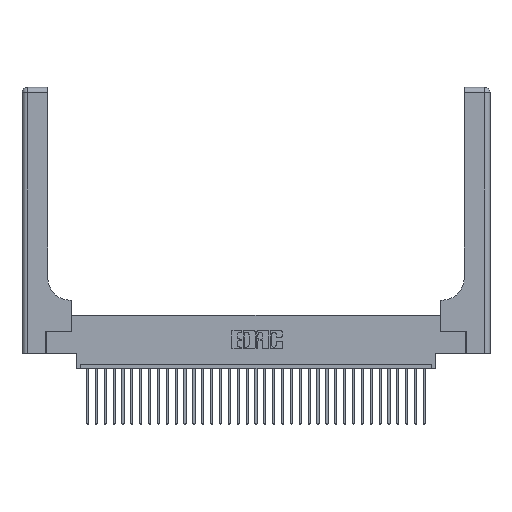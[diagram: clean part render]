
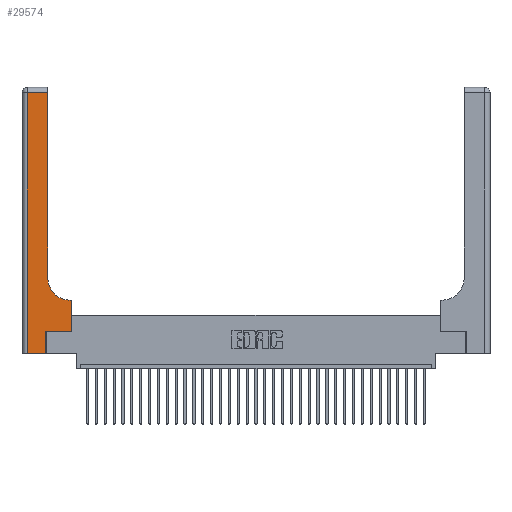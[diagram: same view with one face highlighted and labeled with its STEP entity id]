
A CAD part, top view. The second image highlights one B-rep face of the part: STEP entity #29574.
In plain terms, the highlighted planar face has unit normal (0, 0, 1).
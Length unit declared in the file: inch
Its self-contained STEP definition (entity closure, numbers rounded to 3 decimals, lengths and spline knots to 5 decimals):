
#1807 = VECTOR ( 'NONE', #23549, 39.37008 ) ;
#2154 = VERTEX_POINT ( 'NONE', #17191 ) ;
#2753 = CIRCLE ( 'NONE', #10083, 0.25 ) ;
#4222 = CARTESIAN_POINT ( 'NONE',  ( 0.2915, 3., 0.37 ) ) ;
#4265 = EDGE_CURVE ( 'NONE', #19982, #17829, #9771, .T. ) ;
#4856 = VERTEX_POINT ( 'NONE', #8780 ) ;
#5241 = VECTOR ( 'NONE', #5458, 39.37008 ) ;
#5458 = DIRECTION ( 'NONE',  ( 0., -1., 0. ) ) ;
#6608 = CARTESIAN_POINT ( 'NONE',  ( 0., 3., 0.37 ) ) ;
#6723 = CARTESIAN_POINT ( 'NONE',  ( 0.269, 0., 0.37 ) ) ;
#7131 = FACE_OUTER_BOUND ( 'NONE', #16927, .T. ) ;
#7163 = CARTESIAN_POINT ( 'NONE',  ( 0.269, 0.25, 0.37 ) ) ;
#7577 = VERTEX_POINT ( 'NONE', #15437 ) ;
#8157 = DIRECTION ( 'NONE',  ( 1., 0., 0. ) ) ;
#8568 = LINE ( 'NONE', #16224, #1807 ) ;
#8780 = CARTESIAN_POINT ( 'NONE',  ( 0.06, 2.94, 0.37 ) ) ;
#9764 = EDGE_CURVE ( 'NONE', #7577, #31835, #14838, .T. ) ;
#9771 = LINE ( 'NONE', #4222, #22392 ) ;
#9813 = ORIENTED_EDGE ( 'NONE', *, *, #4265, .T. ) ;
#9881 = ORIENTED_EDGE ( 'NONE', *, *, #16773, .T. ) ;
#10083 = AXIS2_PLACEMENT_3D ( 'NONE', #32426, #24241, #8157 ) ;
#11196 = ORIENTED_EDGE ( 'NONE', *, *, #32418, .T. ) ;
#11605 = VECTOR ( 'NONE', #15889, 39.37008 ) ;
#11642 = CARTESIAN_POINT ( 'NONE',  ( 0.5585, 0.25, 0.37 ) ) ;
#11694 = CARTESIAN_POINT ( 'NONE',  ( 0.5415, 0.6, 0.37 ) ) ;
#12019 = EDGE_CURVE ( 'NONE', #17829, #4856, #26405, .T. ) ;
#12811 = AXIS2_PLACEMENT_3D ( 'NONE', #6608, #15139, #17930 ) ;
#12861 = ORIENTED_EDGE ( 'NONE', *, *, #9764, .T. ) ;
#14224 = LINE ( 'NONE', #33709, #27313 ) ;
#14408 = VERTEX_POINT ( 'NONE', #31009 ) ;
#14838 = LINE ( 'NONE', #7163, #24172 ) ;
#15139 = DIRECTION ( 'NONE',  ( 0., 0., -1. ) ) ;
#15437 = CARTESIAN_POINT ( 'NONE',  ( 0.269, 0.25, 0.37 ) ) ;
#15889 = DIRECTION ( 'NONE',  ( -1., 0., 0. ) ) ;
#15929 = CARTESIAN_POINT ( 'NONE',  ( 0.2915, 0.85, 0.37 ) ) ;
#16224 = CARTESIAN_POINT ( 'NONE',  ( 0.2915, 0.6, 0.37 ) ) ;
#16773 = EDGE_CURVE ( 'NONE', #14408, #25531, #8568, .T. ) ;
#16927 = EDGE_LOOP ( 'NONE', ( #9813, #30972, #29127, #30011, #11196, #12861, #18598, #9881, #34941 ) ) ;
#17075 = VECTOR ( 'NONE', #30479, 39.37008 ) ;
#17191 = CARTESIAN_POINT ( 'NONE',  ( 0.269, 0., 0.37 ) ) ;
#17829 = VERTEX_POINT ( 'NONE', #33732 ) ;
#17930 = DIRECTION ( 'NONE',  ( -1., 0., 0. ) ) ;
#18349 = CARTESIAN_POINT ( 'NONE',  ( 0., 2.94, 0.37 ) ) ;
#18381 = DIRECTION ( 'NONE',  ( 0., 1., 0. ) ) ;
#18598 = ORIENTED_EDGE ( 'NONE', *, *, #21424, .T. ) ;
#19684 = CARTESIAN_POINT ( 'NONE',  ( 0., 0., 0.37 ) ) ;
#19982 = VERTEX_POINT ( 'NONE', #15929 ) ;
#20419 = VERTEX_POINT ( 'NONE', #28090 ) ;
#21424 = EDGE_CURVE ( 'NONE', #31835, #14408, #14224, .T. ) ;
#21638 = CARTESIAN_POINT ( 'NONE',  ( 0.06, 3., 0.37 ) ) ;
#21829 = EDGE_CURVE ( 'NONE', #25531, #19982, #2753, .T. ) ;
#22392 = VECTOR ( 'NONE', #34275, 39.37008 ) ;
#23549 = DIRECTION ( 'NONE',  ( -1., 0., 0. ) ) ;
#24172 = VECTOR ( 'NONE', #28338, 39.37008 ) ;
#24241 = DIRECTION ( 'NONE',  ( 0., 0., -1. ) ) ;
#25509 = DIRECTION ( 'NONE',  ( 1., 0., 0. ) ) ;
#25531 = VERTEX_POINT ( 'NONE', #11694 ) ;
#26405 = LINE ( 'NONE', #18349, #11605 ) ;
#26417 = LINE ( 'NONE', #19684, #30647 ) ;
#27313 = VECTOR ( 'NONE', #18381, 39.37008 ) ;
#28090 = CARTESIAN_POINT ( 'NONE',  ( 0.06, 0., 0.37 ) ) ;
#28338 = DIRECTION ( 'NONE',  ( 1., 0., 0. ) ) ;
#29127 = ORIENTED_EDGE ( 'NONE', *, *, #32615, .T. ) ;
#29574 = ADVANCED_FACE ( 'NONE', ( #7131 ), #31233, .F. ) ;
#30011 = ORIENTED_EDGE ( 'NONE', *, *, #32438, .T. ) ;
#30479 = DIRECTION ( 'NONE',  ( 0., 1., 0. ) ) ;
#30647 = VECTOR ( 'NONE', #25509, 39.37008 ) ;
#30972 = ORIENTED_EDGE ( 'NONE', *, *, #12019, .T. ) ;
#31009 = CARTESIAN_POINT ( 'NONE',  ( 0.5585, 0.6, 0.37 ) ) ;
#31076 = LINE ( 'NONE', #21638, #5241 ) ;
#31233 = PLANE ( 'NONE',  #12811 ) ;
#31835 = VERTEX_POINT ( 'NONE', #11642 ) ;
#32418 = EDGE_CURVE ( 'NONE', #2154, #7577, #33219, .T. ) ;
#32426 = CARTESIAN_POINT ( 'NONE',  ( 0.5415, 0.85, 0.37 ) ) ;
#32438 = EDGE_CURVE ( 'NONE', #20419, #2154, #26417, .T. ) ;
#32615 = EDGE_CURVE ( 'NONE', #4856, #20419, #31076, .T. ) ;
#33219 = LINE ( 'NONE', #6723, #17075 ) ;
#33709 = CARTESIAN_POINT ( 'NONE',  ( 0.5585, 0.25, 0.37 ) ) ;
#33732 = CARTESIAN_POINT ( 'NONE',  ( 0.2915, 2.94, 0.37 ) ) ;
#34275 = DIRECTION ( 'NONE',  ( 0., 1., 0. ) ) ;
#34941 = ORIENTED_EDGE ( 'NONE', *, *, #21829, .T. ) ;
